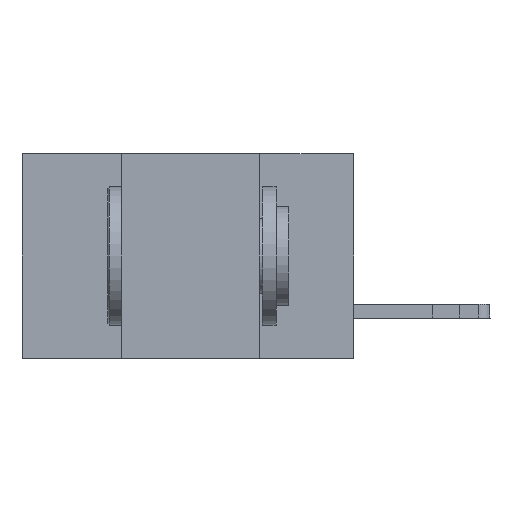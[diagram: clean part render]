
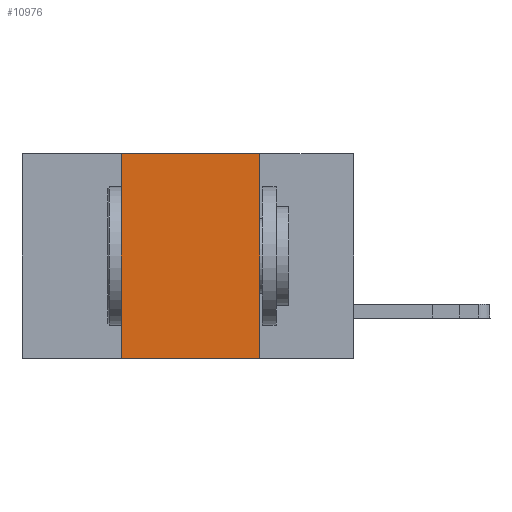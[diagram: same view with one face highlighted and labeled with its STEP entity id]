
A CAD part, left-side view. The second image highlights one B-rep face of the part: STEP entity #10976.
In plain terms, the highlighted planar face has unit normal (-1, 0, 0).
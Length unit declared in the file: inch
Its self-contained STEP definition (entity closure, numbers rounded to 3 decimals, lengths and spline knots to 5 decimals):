
#969 = CARTESIAN_POINT ( 'NONE',  ( 0., 0.42, 0. ) ) ;
#1056 = PLANE ( 'NONE',  #11633 ) ;
#1379 = CARTESIAN_POINT ( 'NONE',  ( 0., 0.42, -0.37 ) ) ;
#1707 = VECTOR ( 'NONE', #4561, 39.37008 ) ;
#1747 = CARTESIAN_POINT ( 'NONE',  ( 0., 0.42, 0. ) ) ;
#3807 = ORIENTED_EDGE ( 'NONE', *, *, #16767, .F. ) ;
#4561 = DIRECTION ( 'NONE',  ( 0., 0., -1. ) ) ;
#4700 = CARTESIAN_POINT ( 'NONE',  ( 0., 0.17, -0.37 ) ) ;
#5513 = VERTEX_POINT ( 'NONE', #4700 ) ;
#5898 = EDGE_CURVE ( 'NONE', #12152, #5513, #20203, .T. ) ;
#5922 = DIRECTION ( 'NONE',  ( 0., -1., 0. ) ) ;
#6040 = LINE ( 'NONE', #6374, #20991 ) ;
#6374 = CARTESIAN_POINT ( 'NONE',  ( 0., 0.6, -0.37 ) ) ;
#6921 = ORIENTED_EDGE ( 'NONE', *, *, #5898, .F. ) ;
#7301 = VECTOR ( 'NONE', #17024, 39.37008 ) ;
#8073 = CARTESIAN_POINT ( 'NONE',  ( 0., 0.6, 0. ) ) ;
#9848 = LINE ( 'NONE', #969, #21353 ) ;
#10245 = CARTESIAN_POINT ( 'NONE',  ( 0., 0.6, 0. ) ) ;
#10976 = ADVANCED_FACE ( 'NONE', ( #20656 ), #1056, .F. ) ;
#11633 = AXIS2_PLACEMENT_3D ( 'NONE', #8073, #20766, #11673 ) ;
#11673 = DIRECTION ( 'NONE',  ( 0., 0., -1. ) ) ;
#12152 = VERTEX_POINT ( 'NONE', #22759 ) ;
#12880 = ORIENTED_EDGE ( 'NONE', *, *, #13973, .T. ) ;
#13279 = VERTEX_POINT ( 'NONE', #1747 ) ;
#13973 = EDGE_CURVE ( 'NONE', #21061, #5513, #6040, .T. ) ;
#14422 = EDGE_CURVE ( 'NONE', #21061, #13279, #9848, .T. ) ;
#15438 = ORIENTED_EDGE ( 'NONE', *, *, #14422, .F. ) ;
#16767 = EDGE_CURVE ( 'NONE', #13279, #12152, #20634, .T. ) ;
#17024 = DIRECTION ( 'NONE',  ( 0., -1., 0. ) ) ;
#20203 = LINE ( 'NONE', #20534, #1707 ) ;
#20534 = CARTESIAN_POINT ( 'NONE',  ( 0., 0.17, 0. ) ) ;
#20634 = LINE ( 'NONE', #10245, #7301 ) ;
#20656 = FACE_OUTER_BOUND ( 'NONE', #21331, .T. ) ;
#20766 = DIRECTION ( 'NONE',  ( 1., 0., 0. ) ) ;
#20991 = VECTOR ( 'NONE', #5922, 39.37008 ) ;
#21061 = VERTEX_POINT ( 'NONE', #1379 ) ;
#21331 = EDGE_LOOP ( 'NONE', ( #6921, #3807, #15438, #12880 ) ) ;
#21353 = VECTOR ( 'NONE', #22329, 39.37008 ) ;
#22329 = DIRECTION ( 'NONE',  ( 0., 0., 1. ) ) ;
#22759 = CARTESIAN_POINT ( 'NONE',  ( 0., 0.17, 0. ) ) ;
